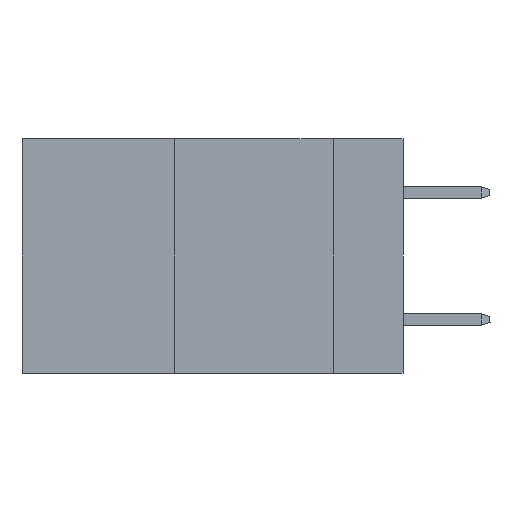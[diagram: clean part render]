
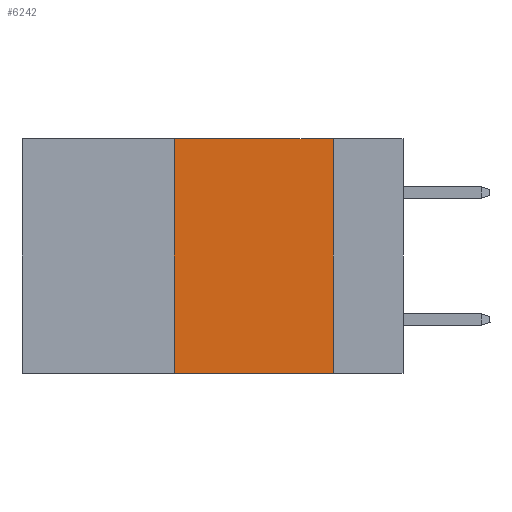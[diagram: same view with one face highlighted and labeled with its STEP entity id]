
A CAD part, left-side view. The second image highlights one B-rep face of the part: STEP entity #6242.
In plain terms, the highlighted planar face has unit normal (-1, 0, 0).
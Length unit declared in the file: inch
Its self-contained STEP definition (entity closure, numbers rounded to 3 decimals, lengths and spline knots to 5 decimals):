
#313 = VECTOR ( 'NONE', #14065, 39.37008 ) ;
#497 = DIRECTION ( 'NONE',  ( 0., 0., 1. ) ) ;
#504 = VERTEX_POINT ( 'NONE', #14020 ) ;
#821 = FACE_OUTER_BOUND ( 'NONE', #7093, .T. ) ;
#1177 = CARTESIAN_POINT ( 'NONE',  ( 0., 0.11, -0.37 ) ) ;
#1508 = EDGE_CURVE ( 'NONE', #504, #6016, #13018, .T. ) ;
#1896 = CARTESIAN_POINT ( 'NONE',  ( 0., 0.6, -0.37 ) ) ;
#2895 = VECTOR ( 'NONE', #497, 39.37008 ) ;
#3537 = ORIENTED_EDGE ( 'NONE', *, *, #14716, .F. ) ;
#4144 = CARTESIAN_POINT ( 'NONE',  ( 0., 0.11, 0. ) ) ;
#4558 = LINE ( 'NONE', #11107, #2895 ) ;
#4616 = CARTESIAN_POINT ( 'NONE',  ( 0., 0.36, 0. ) ) ;
#4803 = VERTEX_POINT ( 'NONE', #4616 ) ;
#5017 = DIRECTION ( 'NONE',  ( 0., -1., 0. ) ) ;
#5019 = DIRECTION ( 'NONE',  ( 0., 0., -1. ) ) ;
#5070 = DIRECTION ( 'NONE',  ( 0., 0., -1. ) ) ;
#5188 = ORIENTED_EDGE ( 'NONE', *, *, #1508, .T. ) ;
#6016 = VERTEX_POINT ( 'NONE', #1177 ) ;
#6242 = ADVANCED_FACE ( 'NONE', ( #821 ), #15574, .F. ) ;
#6521 = CARTESIAN_POINT ( 'NONE',  ( 0., 0.11, 0. ) ) ;
#7093 = EDGE_LOOP ( 'NONE', ( #11027, #14733, #3537, #5188 ) ) ;
#8298 = VECTOR ( 'NONE', #5019, 39.37008 ) ;
#9151 = LINE ( 'NONE', #11727, #14763 ) ;
#10290 = CARTESIAN_POINT ( 'NONE',  ( 0., 0.6, 0. ) ) ;
#10745 = LINE ( 'NONE', #6521, #8298 ) ;
#11027 = ORIENTED_EDGE ( 'NONE', *, *, #15039, .F. ) ;
#11107 = CARTESIAN_POINT ( 'NONE',  ( 0., 0.36, 0. ) ) ;
#11727 = CARTESIAN_POINT ( 'NONE',  ( 0., 0.6, 0. ) ) ;
#12981 = VERTEX_POINT ( 'NONE', #4144 ) ;
#13018 = LINE ( 'NONE', #1896, #313 ) ;
#13676 = EDGE_CURVE ( 'NONE', #4803, #12981, #9151, .T. ) ;
#14020 = CARTESIAN_POINT ( 'NONE',  ( 0., 0.36, -0.37 ) ) ;
#14065 = DIRECTION ( 'NONE',  ( 0., -1., 0. ) ) ;
#14716 = EDGE_CURVE ( 'NONE', #504, #4803, #4558, .T. ) ;
#14733 = ORIENTED_EDGE ( 'NONE', *, *, #13676, .F. ) ;
#14763 = VECTOR ( 'NONE', #5017, 39.37008 ) ;
#15039 = EDGE_CURVE ( 'NONE', #12981, #6016, #10745, .T. ) ;
#15574 = PLANE ( 'NONE',  #16437 ) ;
#16437 = AXIS2_PLACEMENT_3D ( 'NONE', #10290, #17185, #5070 ) ;
#17185 = DIRECTION ( 'NONE',  ( 1., 0., 0. ) ) ;
